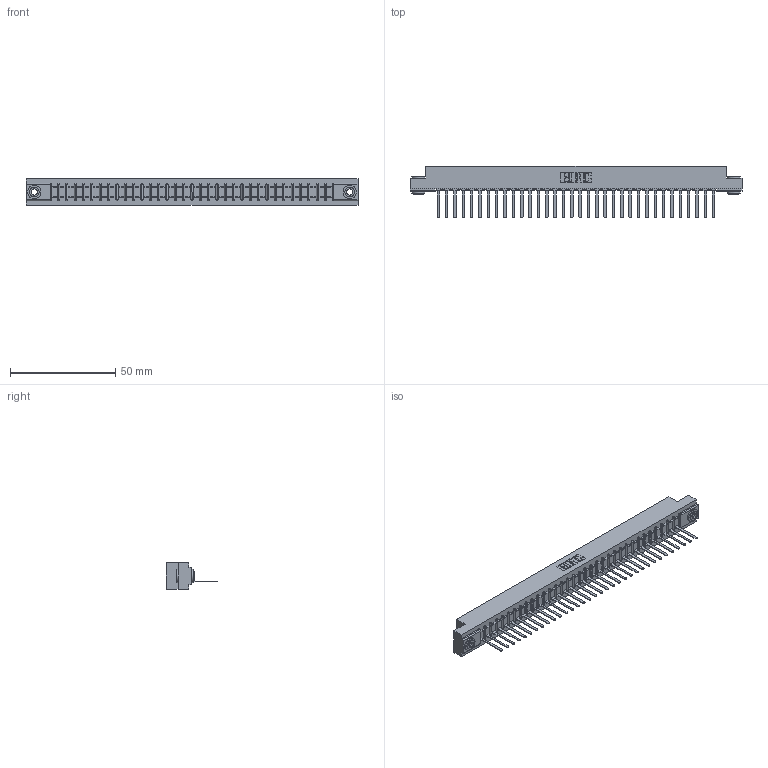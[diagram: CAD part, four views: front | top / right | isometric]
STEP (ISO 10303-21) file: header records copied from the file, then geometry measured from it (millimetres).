
FILE_DESCRIPTION (( 'STEP AP203' ), '1' );
FILE_NAME ('307-034-441-103.STEP', '2020-09-28T21:24:51', ( '' ), ( '' ), 'SwSTEP 2.0', 'SolidWorks 2020', '' );
FILE_SCHEMA (( 'CONFIG_CONTROL_DESIGN' ));
Length unit declared in the file: inch
Products named in the file (4): 345-250-002_345-250-002-102; 307-034-441-103; 307 Part_.156 Dia Mounting Holes; 307-290-002_541
Assembly tree (37 placements, depth 2):
  307-034-441-103
    307 Part_.156 Dia Mounting Holes
    307-290-002_541  x34
    345-250-002_345-250-002-102  x2
Bounding box: 157.73 x 24.59 x 12.7 mm (x, y, z)
Volume: 16917.1 mm3; surface area: 21962.5 mm2
Topology: 37 solids, 37 shells, 2721 faces, 8323 edges, 5450 vertices
Faces by surface type: plane 1624, cylinder 1019, sphere 70, cone 8
Entity records: 31917 total; most frequent: CARTESIAN_POINT 5361, ORIENTED_EDGE 5342, DIRECTION 5227, EDGE_CURVE 2671, LINE 2035, VECTOR 2035, VERTEX_POINT 1730, AXIS2_PLACEMENT_3D 1596
